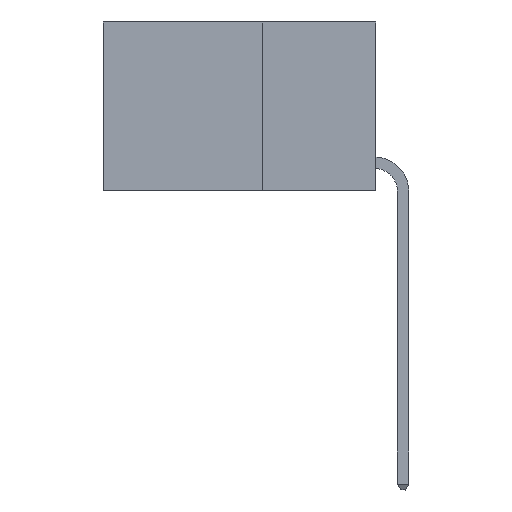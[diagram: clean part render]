
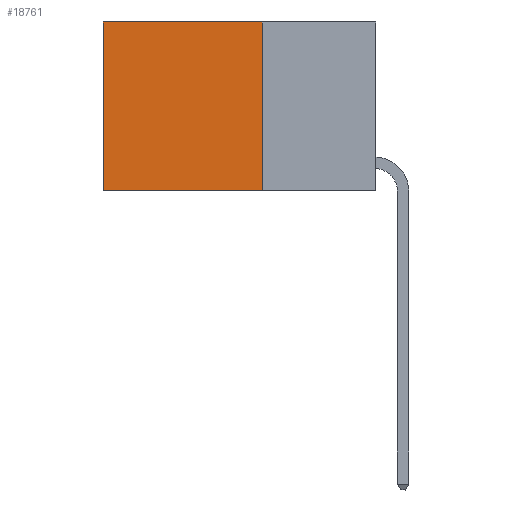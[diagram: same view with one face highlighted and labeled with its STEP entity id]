
A CAD part, left-side view. The second image highlights one B-rep face of the part: STEP entity #18761.
In plain terms, the highlighted planar face has unit normal (-1, 0, 0).
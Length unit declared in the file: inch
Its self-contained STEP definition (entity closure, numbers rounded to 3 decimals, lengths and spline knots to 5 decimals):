
#1233 = VECTOR ( 'NONE', #22467, 39.37008 ) ;
#1911 = CARTESIAN_POINT ( 'NONE',  ( 0.2625, 0.25, 0. ) ) ;
#2143 = ORIENTED_EDGE ( 'NONE', *, *, #10887, .F. ) ;
#3398 = CARTESIAN_POINT ( 'NONE',  ( 0.2625, 0.25, 0. ) ) ;
#4303 = DIRECTION ( 'NONE',  ( 0., 0., -1. ) ) ;
#4601 = EDGE_CURVE ( 'NONE', #9480, #7050, #18724, .T. ) ;
#5703 = ORIENTED_EDGE ( 'NONE', *, *, #18888, .F. ) ;
#5810 = PLANE ( 'NONE',  #14333 ) ;
#7017 = LINE ( 'NONE', #15915, #1233 ) ;
#7050 = VERTEX_POINT ( 'NONE', #20246 ) ;
#7078 = ORIENTED_EDGE ( 'NONE', *, *, #7488, .T. ) ;
#7182 = VECTOR ( 'NONE', #9894, 39.37008 ) ;
#7488 = EDGE_CURVE ( 'NONE', #7050, #12274, #23334, .T. ) ;
#9157 = EDGE_LOOP ( 'NONE', ( #7078, #2143, #5703, #23342 ) ) ;
#9480 = VERTEX_POINT ( 'NONE', #19744 ) ;
#9894 = DIRECTION ( 'NONE',  ( 0., 1., 0. ) ) ;
#10161 = DIRECTION ( 'NONE',  ( 0., 0., -1. ) ) ;
#10724 = CARTESIAN_POINT ( 'NONE',  ( 0.2625, 0.6, 0. ) ) ;
#10887 = EDGE_CURVE ( 'NONE', #27777, #12274, #7017, .T. ) ;
#11096 = VECTOR ( 'NONE', #4303, 39.37008 ) ;
#12274 = VERTEX_POINT ( 'NONE', #17574 ) ;
#12707 = DIRECTION ( 'NONE',  ( 0., 0., -1. ) ) ;
#14333 = AXIS2_PLACEMENT_3D ( 'NONE', #20999, #23185, #10161 ) ;
#15503 = LINE ( 'NONE', #1911, #26289 ) ;
#15626 = CARTESIAN_POINT ( 'NONE',  ( 0.2625, 0.25, -0.37 ) ) ;
#15915 = CARTESIAN_POINT ( 'NONE',  ( 0.2625, 0.25, -0.37 ) ) ;
#17574 = CARTESIAN_POINT ( 'NONE',  ( 0.2625, 0.6, -0.37 ) ) ;
#18216 = FACE_OUTER_BOUND ( 'NONE', #9157, .T. ) ;
#18724 = LINE ( 'NONE', #3398, #7182 ) ;
#18761 = ADVANCED_FACE ( 'NONE', ( #18216 ), #5810, .F. ) ;
#18888 = EDGE_CURVE ( 'NONE', #9480, #27777, #15503, .T. ) ;
#19744 = CARTESIAN_POINT ( 'NONE',  ( 0.2625, 0.25, 0. ) ) ;
#20246 = CARTESIAN_POINT ( 'NONE',  ( 0.2625, 0.6, 0. ) ) ;
#20999 = CARTESIAN_POINT ( 'NONE',  ( 0.2625, 0.25, 0. ) ) ;
#22467 = DIRECTION ( 'NONE',  ( 0., 1., 0. ) ) ;
#23185 = DIRECTION ( 'NONE',  ( 1., 0., 0. ) ) ;
#23334 = LINE ( 'NONE', #10724, #11096 ) ;
#23342 = ORIENTED_EDGE ( 'NONE', *, *, #4601, .T. ) ;
#26289 = VECTOR ( 'NONE', #12707, 39.37008 ) ;
#27777 = VERTEX_POINT ( 'NONE', #15626 ) ;
